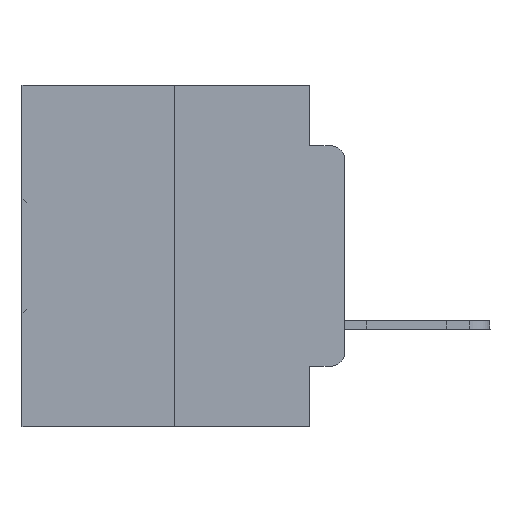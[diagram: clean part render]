
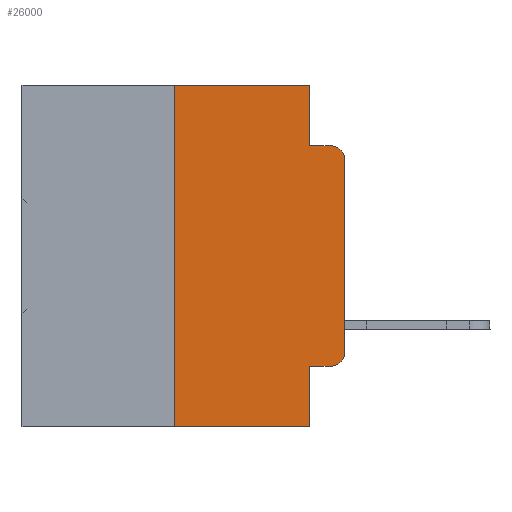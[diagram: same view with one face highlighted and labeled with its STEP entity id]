
A CAD part, left-side view. The second image highlights one B-rep face of the part: STEP entity #26000.
In plain terms, the highlighted planar face has unit normal (-1, 0, 0).
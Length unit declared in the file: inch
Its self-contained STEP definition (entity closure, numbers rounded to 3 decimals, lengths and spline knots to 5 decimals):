
#86 = LINE ( 'NONE', #10953, #10258 ) ;
#217 = PLANE ( 'NONE',  #25244 ) ;
#653 = DIRECTION ( 'NONE',  ( 0., 0., -1. ) ) ;
#1037 = VERTEX_POINT ( 'NONE', #13029 ) ;
#1045 = VECTOR ( 'NONE', #16928, 39.37008 ) ;
#1883 = LINE ( 'NONE', #13538, #16357 ) ;
#1958 = AXIS2_PLACEMENT_3D ( 'NONE', #14271, #11638, #4035 ) ;
#2343 = EDGE_CURVE ( 'NONE', #3779, #1037, #9531, .T. ) ;
#3453 = CARTESIAN_POINT ( 'NONE',  ( 0., 0.051, -0.0885 ) ) ;
#3726 = VERTEX_POINT ( 'NONE', #13426 ) ;
#3779 = VERTEX_POINT ( 'NONE', #10920 ) ;
#3929 = VERTEX_POINT ( 'NONE', #24127 ) ;
#4035 = DIRECTION ( 'NONE',  ( 0., 0., -1. ) ) ;
#4318 = LINE ( 'NONE', #3453, #21119 ) ;
#5131 = LINE ( 'NONE', #17668, #28919 ) ;
#5164 = EDGE_CURVE ( 'NONE', #29582, #12922, #30353, .T. ) ;
#5746 = ORIENTED_EDGE ( 'NONE', *, *, #2343, .F. ) ;
#5964 = VERTEX_POINT ( 'NONE', #14263 ) ;
#6064 = DIRECTION ( 'NONE',  ( 0., -1., 0. ) ) ;
#6091 = ORIENTED_EDGE ( 'NONE', *, *, #31666, .T. ) ;
#6405 = EDGE_CURVE ( 'NONE', #3929, #1037, #28387, .T. ) ;
#6748 = DIRECTION ( 'NONE',  ( 0., 0., -1. ) ) ;
#7819 = FACE_OUTER_BOUND ( 'NONE', #14823, .T. ) ;
#8037 = ORIENTED_EDGE ( 'NONE', *, *, #30951, .F. ) ;
#9531 = LINE ( 'NONE', #26292, #24758 ) ;
#10258 = VECTOR ( 'NONE', #6064, 39.37008 ) ;
#10662 = EDGE_CURVE ( 'NONE', #5964, #12922, #4318, .T. ) ;
#10920 = CARTESIAN_POINT ( 'NONE',  ( 0., 0.051, -0.4115 ) ) ;
#10953 = CARTESIAN_POINT ( 'NONE',  ( 0., 0.051, -0.4115 ) ) ;
#11298 = EDGE_CURVE ( 'NONE', #19986, #22819, #1883, .T. ) ;
#11638 = DIRECTION ( 'NONE',  ( -1., 0., 0. ) ) ;
#12198 = ORIENTED_EDGE ( 'NONE', *, *, #10662, .F. ) ;
#12602 = EDGE_CURVE ( 'NONE', #26376, #3726, #27178, .T. ) ;
#12922 = VERTEX_POINT ( 'NONE', #23413 ) ;
#13029 = CARTESIAN_POINT ( 'NONE',  ( 0., 0.051, -0.5 ) ) ;
#13426 = CARTESIAN_POINT ( 'NONE',  ( 0., 0., -0.3915 ) ) ;
#13538 = CARTESIAN_POINT ( 'NONE',  ( 0., 0.473, 0. ) ) ;
#14256 = ORIENTED_EDGE ( 'NONE', *, *, #29760, .T. ) ;
#14263 = CARTESIAN_POINT ( 'NONE',  ( 0., 0.051, -0.0885 ) ) ;
#14271 = CARTESIAN_POINT ( 'NONE',  ( 0., 0.02, -0.3915 ) ) ;
#14489 = DIRECTION ( 'NONE',  ( 0., 0., 1. ) ) ;
#14823 = EDGE_LOOP ( 'NONE', ( #6091, #23993, #12198, #8037, #20599, #32099, #16502, #5746, #14256, #25296 ) ) ;
#15981 = DIRECTION ( 'NONE',  ( 0., -1., 0. ) ) ;
#16357 = VECTOR ( 'NONE', #28265, 39.37008 ) ;
#16502 = ORIENTED_EDGE ( 'NONE', *, *, #6405, .T. ) ;
#16928 = DIRECTION ( 'NONE',  ( 0., -1., 0. ) ) ;
#17524 = CARTESIAN_POINT ( 'NONE',  ( 0., 0., -0.1085 ) ) ;
#17668 = CARTESIAN_POINT ( 'NONE',  ( 0., 0.051, 0. ) ) ;
#18111 = DIRECTION ( 'NONE',  ( 0., 0., -1. ) ) ;
#18266 = EDGE_CURVE ( 'NONE', #3929, #19986, #31975, .T. ) ;
#18431 = CARTESIAN_POINT ( 'NONE',  ( 0., 0.051, 0. ) ) ;
#19216 = CARTESIAN_POINT ( 'NONE',  ( 0., 0.02, -0.1085 ) ) ;
#19986 = VERTEX_POINT ( 'NONE', #28492 ) ;
#20599 = ORIENTED_EDGE ( 'NONE', *, *, #11298, .F. ) ;
#21083 = VECTOR ( 'NONE', #14489, 39.37008 ) ;
#21119 = VECTOR ( 'NONE', #15981, 39.37008 ) ;
#21727 = DIRECTION ( 'NONE',  ( -1., 0., 0. ) ) ;
#21842 = AXIS2_PLACEMENT_3D ( 'NONE', #19216, #21727, #6748 ) ;
#22760 = CARTESIAN_POINT ( 'NONE',  ( 0., 0.473, 0. ) ) ;
#22789 = CARTESIAN_POINT ( 'NONE',  ( 0., 0., 0. ) ) ;
#22819 = VERTEX_POINT ( 'NONE', #18431 ) ;
#23413 = CARTESIAN_POINT ( 'NONE',  ( 0., 0.02, -0.0885 ) ) ;
#23585 = VECTOR ( 'NONE', #25473, 39.37008 ) ;
#23928 = DIRECTION ( 'NONE',  ( 0., 0., -1. ) ) ;
#23993 = ORIENTED_EDGE ( 'NONE', *, *, #5164, .T. ) ;
#24127 = CARTESIAN_POINT ( 'NONE',  ( 0., 0.25, -0.5 ) ) ;
#24758 = VECTOR ( 'NONE', #23928, 39.37008 ) ;
#25244 = AXIS2_PLACEMENT_3D ( 'NONE', #22760, #25654, #653 ) ;
#25296 = ORIENTED_EDGE ( 'NONE', *, *, #12602, .T. ) ;
#25473 = DIRECTION ( 'NONE',  ( 0., 0., 1. ) ) ;
#25654 = DIRECTION ( 'NONE',  ( 1., 0., 0. ) ) ;
#26000 = ADVANCED_FACE ( 'NONE', ( #7819 ), #217, .F. ) ;
#26292 = CARTESIAN_POINT ( 'NONE',  ( 0., 0.051, 0. ) ) ;
#26376 = VERTEX_POINT ( 'NONE', #32304 ) ;
#27178 = CIRCLE ( 'NONE', #1958, 0.02 ) ;
#28265 = DIRECTION ( 'NONE',  ( 0., -1., 0. ) ) ;
#28387 = LINE ( 'NONE', #31861, #1045 ) ;
#28492 = CARTESIAN_POINT ( 'NONE',  ( 0., 0.25, 0. ) ) ;
#28919 = VECTOR ( 'NONE', #18111, 39.37008 ) ;
#29419 = CARTESIAN_POINT ( 'NONE',  ( 0., 0.25, 0. ) ) ;
#29582 = VERTEX_POINT ( 'NONE', #17524 ) ;
#29760 = EDGE_CURVE ( 'NONE', #3779, #26376, #86, .T. ) ;
#30169 = LINE ( 'NONE', #22789, #23585 ) ;
#30353 = CIRCLE ( 'NONE', #21842, 0.02 ) ;
#30951 = EDGE_CURVE ( 'NONE', #22819, #5964, #5131, .T. ) ;
#31666 = EDGE_CURVE ( 'NONE', #3726, #29582, #30169, .T. ) ;
#31861 = CARTESIAN_POINT ( 'NONE',  ( 0., 0.473, -0.5 ) ) ;
#31975 = LINE ( 'NONE', #29419, #21083 ) ;
#32099 = ORIENTED_EDGE ( 'NONE', *, *, #18266, .F. ) ;
#32304 = CARTESIAN_POINT ( 'NONE',  ( 0., 0.02, -0.4115 ) ) ;
